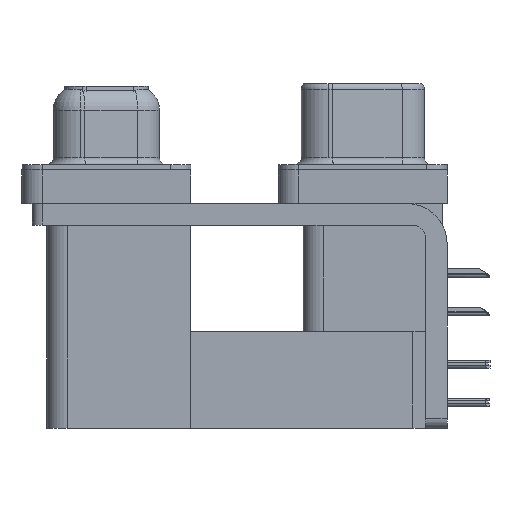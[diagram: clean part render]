
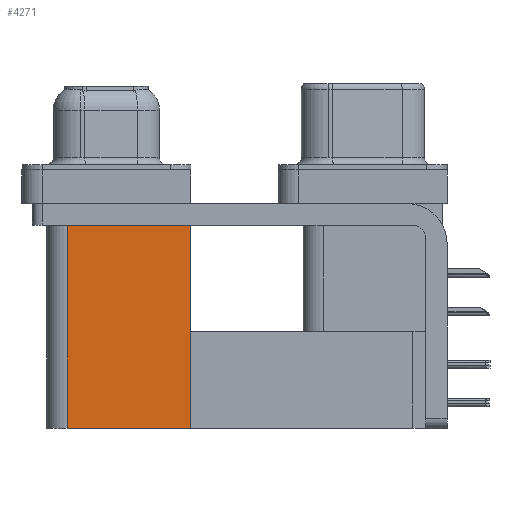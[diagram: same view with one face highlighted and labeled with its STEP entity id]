
A CAD part, left-side view. The second image highlights one B-rep face of the part: STEP entity #4271.
In plain terms, the highlighted planar face has unit normal (-1, 0, 0).
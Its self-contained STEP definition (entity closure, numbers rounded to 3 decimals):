
#261 = DIRECTION ( 'NONE',  ( 0., 1., 0. ) ) ;
#4271 = ADVANCED_FACE ( 'NONE', ( #37842 ), #5212, .F. ) ;
#5212 = PLANE ( 'NONE',  #45123 ) ;
#5911 = ORIENTED_EDGE ( 'NONE', *, *, #42670, .T. ) ;
#13950 = CARTESIAN_POINT ( 'NONE',  ( 3.7, 12.775, -19.2 ) ) ;
#16153 = DIRECTION ( 'NONE',  ( 0., 0., 1. ) ) ;
#16453 = CARTESIAN_POINT ( 'NONE',  ( 3.7, 12.775, -19.2 ) ) ;
#20123 = VECTOR ( 'NONE', #40038, 1000. ) ;
#20393 = CARTESIAN_POINT ( 'NONE',  ( 3.7, 12.775, -2.5 ) ) ;
#23888 = VERTEX_POINT ( 'NONE', #44292 ) ;
#24698 = EDGE_LOOP ( 'NONE', ( #29648, #32777, #43967, #5911 ) ) ;
#25224 = CARTESIAN_POINT ( 'NONE',  ( 3.7, 12.775, -19.2 ) ) ;
#26120 = CARTESIAN_POINT ( 'NONE',  ( 3.7, 12.775, -2.5 ) ) ;
#27196 = VERTEX_POINT ( 'NONE', #43198 ) ;
#29109 = DIRECTION ( 'NONE',  ( 0., 0., -1. ) ) ;
#29648 = ORIENTED_EDGE ( 'NONE', *, *, #41380, .T. ) ;
#30548 = CARTESIAN_POINT ( 'NONE',  ( 3.7, 21.975, -19.2 ) ) ;
#31056 = DIRECTION ( 'NONE',  ( 0., 0., 1. ) ) ;
#32134 = VECTOR ( 'NONE', #16153, 1000. ) ;
#32540 = VECTOR ( 'NONE', #261, 1000. ) ;
#32777 = ORIENTED_EDGE ( 'NONE', *, *, #47232, .F. ) ;
#35129 = EDGE_CURVE ( 'NONE', #52253, #23888, #36373, .T. ) ;
#36068 = LINE ( 'NONE', #20393, #20123 ) ;
#36340 = LINE ( 'NONE', #40564, #32134 ) ;
#36373 = LINE ( 'NONE', #25224, #32540 ) ;
#36892 = VERTEX_POINT ( 'NONE', #26120 ) ;
#37842 = FACE_OUTER_BOUND ( 'NONE', #24698, .T. ) ;
#38208 = VECTOR ( 'NONE', #31056, 1000. ) ;
#40038 = DIRECTION ( 'NONE',  ( 0., 1., 0. ) ) ;
#40564 = CARTESIAN_POINT ( 'NONE',  ( 3.7, 12.775, -19.2 ) ) ;
#41380 = EDGE_CURVE ( 'NONE', #36892, #27196, #36068, .T. ) ;
#42670 = EDGE_CURVE ( 'NONE', #52253, #36892, #36340, .T. ) ;
#43198 = CARTESIAN_POINT ( 'NONE',  ( 3.7, 21.975, -2.5 ) ) ;
#43967 = ORIENTED_EDGE ( 'NONE', *, *, #35129, .F. ) ;
#44292 = CARTESIAN_POINT ( 'NONE',  ( 3.7, 21.975, -19.2 ) ) ;
#45123 = AXIS2_PLACEMENT_3D ( 'NONE', #13950, #49753, #29109 ) ;
#47232 = EDGE_CURVE ( 'NONE', #23888, #27196, #51446, .T. ) ;
#49753 = DIRECTION ( 'NONE',  ( 1., 0., 0. ) ) ;
#51446 = LINE ( 'NONE', #30548, #38208 ) ;
#52253 = VERTEX_POINT ( 'NONE', #16453 ) ;
